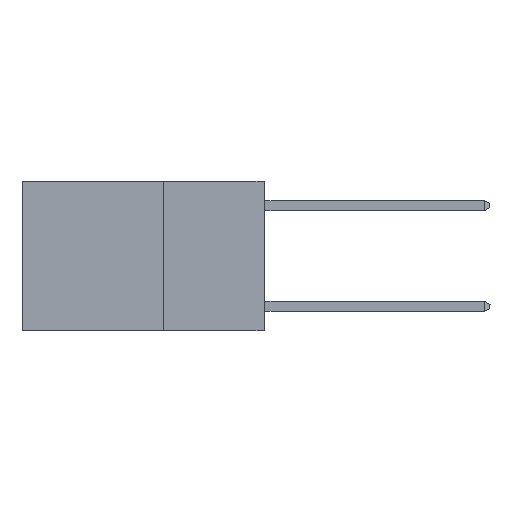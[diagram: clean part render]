
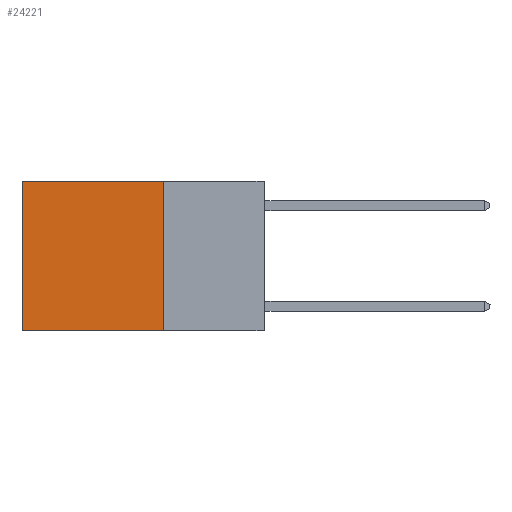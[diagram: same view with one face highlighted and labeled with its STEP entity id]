
A CAD part, left-side view. The second image highlights one B-rep face of the part: STEP entity #24221.
In plain terms, the highlighted planar face has unit normal (-1, 0, 0).
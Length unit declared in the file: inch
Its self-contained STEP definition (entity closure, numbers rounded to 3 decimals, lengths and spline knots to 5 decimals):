
#15 = VECTOR ( 'NONE', #19505, 39.37008 ) ;
#347 = CARTESIAN_POINT ( 'NONE',  ( 0.2625, 0.25, 0. ) ) ;
#764 = LINE ( 'NONE', #17211, #15 ) ;
#1570 = ORIENTED_EDGE ( 'NONE', *, *, #29504, .T. ) ;
#2203 = VERTEX_POINT ( 'NONE', #29027 ) ;
#2272 = EDGE_CURVE ( 'NONE', #18470, #16117, #11407, .T. ) ;
#4311 = ORIENTED_EDGE ( 'NONE', *, *, #16111, .T. ) ;
#5515 = CARTESIAN_POINT ( 'NONE',  ( 0.2625, 0.25, -0.37 ) ) ;
#5609 = CARTESIAN_POINT ( 'NONE',  ( 0.2625, 0.6, 0. ) ) ;
#7632 = CARTESIAN_POINT ( 'NONE',  ( 0.2625, 0.25, 0. ) ) ;
#8501 = CARTESIAN_POINT ( 'NONE',  ( 0.2625, 0.25, 0. ) ) ;
#8633 = AXIS2_PLACEMENT_3D ( 'NONE', #7632, #23869, #9999 ) ;
#9999 = DIRECTION ( 'NONE',  ( 0., 0., -1. ) ) ;
#11081 = FACE_OUTER_BOUND ( 'NONE', #14384, .T. ) ;
#11145 = EDGE_CURVE ( 'NONE', #16117, #2203, #15044, .T. ) ;
#11407 = LINE ( 'NONE', #8501, #16824 ) ;
#14384 = EDGE_LOOP ( 'NONE', ( #1570, #25570, #14626, #4311 ) ) ;
#14626 = ORIENTED_EDGE ( 'NONE', *, *, #2272, .F. ) ;
#15044 = LINE ( 'NONE', #16582, #21147 ) ;
#16111 = EDGE_CURVE ( 'NONE', #18470, #25205, #764, .T. ) ;
#16117 = VERTEX_POINT ( 'NONE', #5515 ) ;
#16582 = CARTESIAN_POINT ( 'NONE',  ( 0.2625, 0.25, -0.37 ) ) ;
#16824 = VECTOR ( 'NONE', #27009, 39.37008 ) ;
#17211 = CARTESIAN_POINT ( 'NONE',  ( 0.2625, 0.25, 0. ) ) ;
#17290 = DIRECTION ( 'NONE',  ( 0., 0., -1. ) ) ;
#17917 = VECTOR ( 'NONE', #17290, 39.37008 ) ;
#18470 = VERTEX_POINT ( 'NONE', #347 ) ;
#19505 = DIRECTION ( 'NONE',  ( 0., 1., 0. ) ) ;
#19676 = CARTESIAN_POINT ( 'NONE',  ( 0.2625, 0.6, 0. ) ) ;
#21147 = VECTOR ( 'NONE', #28039, 39.37008 ) ;
#21541 = PLANE ( 'NONE',  #8633 ) ;
#23869 = DIRECTION ( 'NONE',  ( 1., 0., 0. ) ) ;
#24221 = ADVANCED_FACE ( 'NONE', ( #11081 ), #21541, .F. ) ;
#25205 = VERTEX_POINT ( 'NONE', #5609 ) ;
#25570 = ORIENTED_EDGE ( 'NONE', *, *, #11145, .F. ) ;
#27009 = DIRECTION ( 'NONE',  ( 0., 0., -1. ) ) ;
#28039 = DIRECTION ( 'NONE',  ( 0., 1., 0. ) ) ;
#28376 = LINE ( 'NONE', #19676, #17917 ) ;
#29027 = CARTESIAN_POINT ( 'NONE',  ( 0.2625, 0.6, -0.37 ) ) ;
#29504 = EDGE_CURVE ( 'NONE', #25205, #2203, #28376, .T. ) ;
